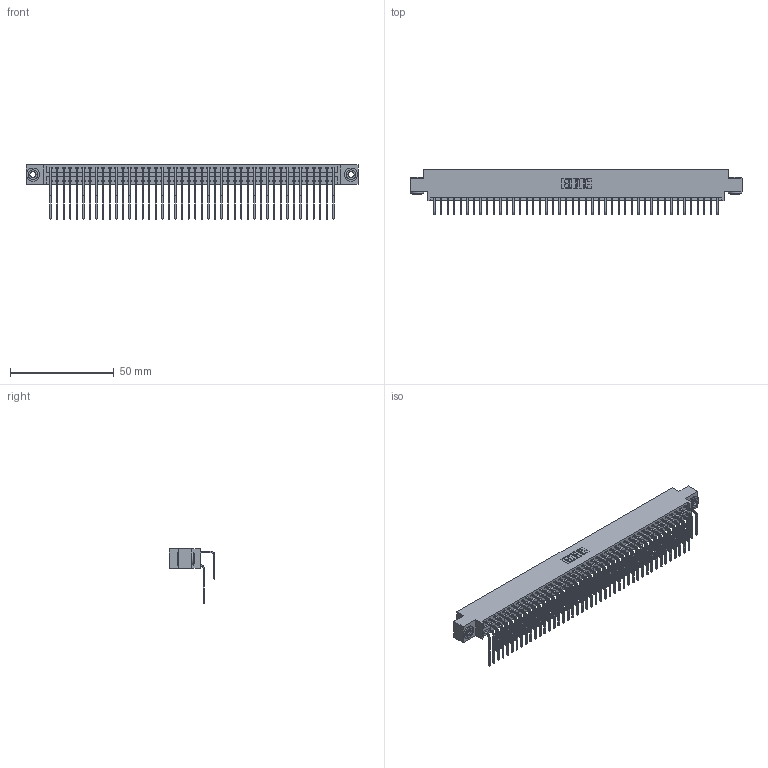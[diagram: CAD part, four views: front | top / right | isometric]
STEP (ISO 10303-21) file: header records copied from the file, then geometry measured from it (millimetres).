
FILE_DESCRIPTION (( 'STEP AP203' ), '1' );
FILE_NAME ('396-088-558-803.STEP', '2018-09-10T06:55:57', ( '' ), ( '' ), 'SwSTEP 2.0', 'SolidWorks 2016', '' );
FILE_SCHEMA (( 'CONFIG_CONTROL_DESIGN' ));
Length unit declared in the file: inch
Products named in the file (5): 346 Part_0.170 Offset - 0.156 Dia-TH; 345-292-001_558 559 Tail - 1; 345-292-001_558 Tail - 2; 345-250-002_345-250-002-102; 396-088-558-803
Assembly tree (91 placements, depth 2):
  396-088-558-803
    346 Part_0.170 Offset - 0.156 Dia-TH
    345-292-001_558 559 Tail - 1  x44
    345-292-001_558 Tail - 2  x44
    345-250-002_345-250-002-102  x2
Bounding box: 160.27 x 22.16 x 26.16 mm (x, y, z)
Volume: 16016.7 mm3; surface area: 24876.6 mm2
Topology: 91 solids, 91 shells, 4916 faces, 14585 edges, 9602 vertices
Faces by surface type: plane 3346, cylinder 1562, cone 8
Entity records: 31012 total; most frequent: CARTESIAN_POINT 5138, ORIENTED_EDGE 5014, DIRECTION 4581, EDGE_CURVE 2507, LINE 2135, VECTOR 2135, VERTEX_POINT 1666, AXIS2_PLACEMENT_3D 1223
